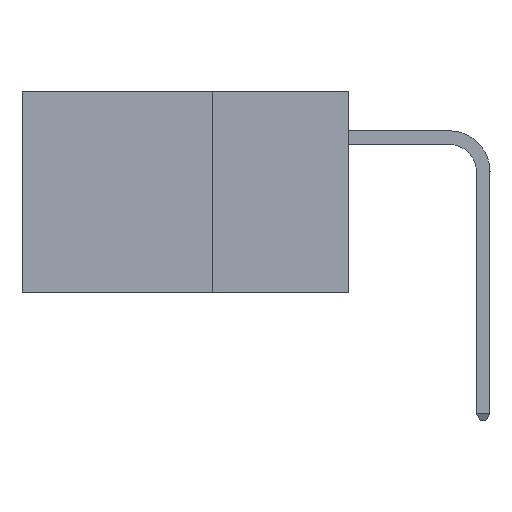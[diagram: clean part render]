
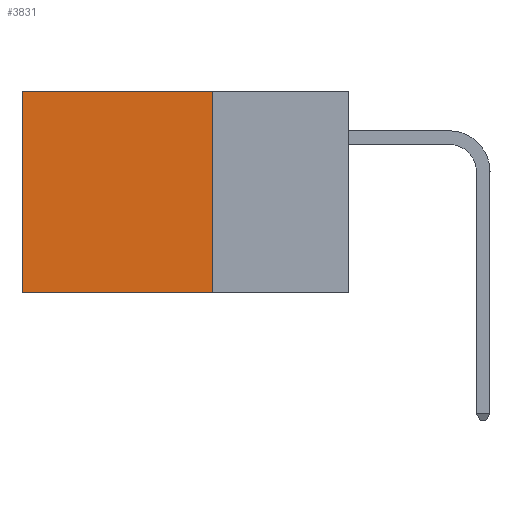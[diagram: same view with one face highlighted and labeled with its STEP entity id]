
A CAD part, left-side view. The second image highlights one B-rep face of the part: STEP entity #3831.
In plain terms, the highlighted planar face has unit normal (-1, 0, 0).
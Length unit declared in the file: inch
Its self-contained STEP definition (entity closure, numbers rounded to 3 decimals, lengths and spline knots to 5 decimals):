
#433 = VERTEX_POINT ( 'NONE', #27128 ) ;
#565 = LINE ( 'NONE', #39594, #30098 ) ;
#1183 = CARTESIAN_POINT ( 'NONE',  ( 0.2875, 0.6, 0. ) ) ;
#1900 = ORIENTED_EDGE ( 'NONE', *, *, #35695, .T. ) ;
#3121 = VERTEX_POINT ( 'NONE', #19874 ) ;
#3752 = AXIS2_PLACEMENT_3D ( 'NONE', #47294, #35974, #13152 ) ;
#3831 = ADVANCED_FACE ( 'NONE', ( #23436 ), #9263, .F. ) ;
#5305 = LINE ( 'NONE', #1183, #35859 ) ;
#9263 = PLANE ( 'NONE',  #3752 ) ;
#10714 = CARTESIAN_POINT ( 'NONE',  ( 0.2875, 0.25, -0.37 ) ) ;
#12057 = ORIENTED_EDGE ( 'NONE', *, *, #17586, .F. ) ;
#12352 = VERTEX_POINT ( 'NONE', #29204 ) ;
#12502 = CARTESIAN_POINT ( 'NONE',  ( 0.2875, 0.25, 0. ) ) ;
#12630 = ORIENTED_EDGE ( 'NONE', *, *, #23502, .T. ) ;
#12887 = EDGE_LOOP ( 'NONE', ( #1900, #24840, #12057, #12630 ) ) ;
#13152 = DIRECTION ( 'NONE',  ( 0., 0., -1. ) ) ;
#15297 = EDGE_CURVE ( 'NONE', #433, #3121, #43364, .T. ) ;
#16380 = DIRECTION ( 'NONE',  ( 0., 0., -1. ) ) ;
#17586 = EDGE_CURVE ( 'NONE', #30431, #433, #37567, .T. ) ;
#19874 = CARTESIAN_POINT ( 'NONE',  ( 0.2875, 0.6, -0.37 ) ) ;
#23436 = FACE_OUTER_BOUND ( 'NONE', #12887, .T. ) ;
#23502 = EDGE_CURVE ( 'NONE', #30431, #12352, #565, .T. ) ;
#24276 = DIRECTION ( 'NONE',  ( 0., 0., -1. ) ) ;
#24840 = ORIENTED_EDGE ( 'NONE', *, *, #15297, .F. ) ;
#27128 = CARTESIAN_POINT ( 'NONE',  ( 0.2875, 0.25, -0.37 ) ) ;
#27468 = VECTOR ( 'NONE', #16380, 39.37008 ) ;
#29204 = CARTESIAN_POINT ( 'NONE',  ( 0.2875, 0.6, 0. ) ) ;
#30098 = VECTOR ( 'NONE', #47257, 39.37008 ) ;
#30431 = VERTEX_POINT ( 'NONE', #31576 ) ;
#31576 = CARTESIAN_POINT ( 'NONE',  ( 0.2875, 0.25, 0. ) ) ;
#34469 = VECTOR ( 'NONE', #37394, 39.37008 ) ;
#35695 = EDGE_CURVE ( 'NONE', #12352, #3121, #5305, .T. ) ;
#35859 = VECTOR ( 'NONE', #24276, 39.37008 ) ;
#35974 = DIRECTION ( 'NONE',  ( 1., 0., 0. ) ) ;
#37394 = DIRECTION ( 'NONE',  ( 0., 1., 0. ) ) ;
#37567 = LINE ( 'NONE', #12502, #27468 ) ;
#39594 = CARTESIAN_POINT ( 'NONE',  ( 0.2875, 0.25, 0. ) ) ;
#43364 = LINE ( 'NONE', #10714, #34469 ) ;
#47257 = DIRECTION ( 'NONE',  ( 0., 1., 0. ) ) ;
#47294 = CARTESIAN_POINT ( 'NONE',  ( 0.2875, 0.25, 0. ) ) ;
